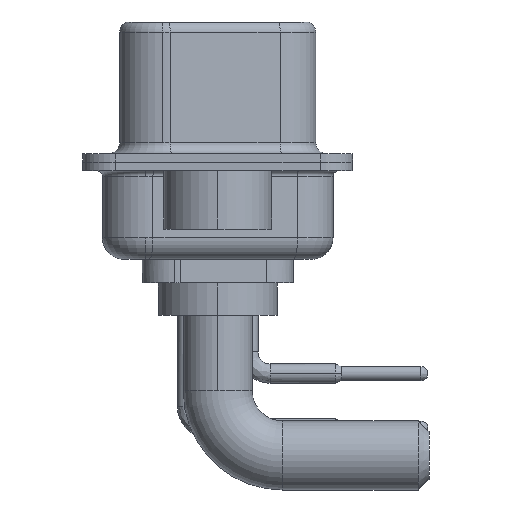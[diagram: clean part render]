
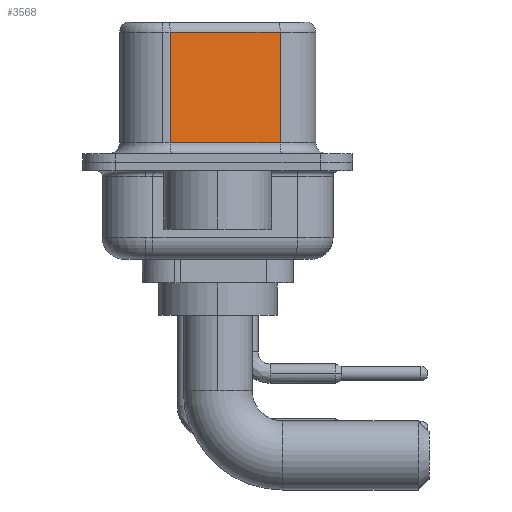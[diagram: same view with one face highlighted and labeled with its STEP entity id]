
A CAD part, left-side view. The second image highlights one B-rep face of the part: STEP entity #3568.
In plain terms, the highlighted planar face has unit normal (-0.985, -0.174, 0).
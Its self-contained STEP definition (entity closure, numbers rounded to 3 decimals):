
#472 = LINE ( 'NONE', #6943, #4627 ) ;
#768 = CARTESIAN_POINT ( 'NONE',  ( 4.555, -2.897, 0.9 ) ) ;
#1092 = EDGE_CURVE ( 'NONE', #7375, #6621, #2627, .T. ) ;
#1129 = EDGE_CURVE ( 'NONE', #11883, #6621, #8667, .T. ) ;
#2255 = EDGE_CURVE ( 'NONE', #7375, #4635, #472, .T. ) ;
#2420 = DIRECTION ( 'NONE',  ( 0.174, -0.985, 0. ) ) ;
#2627 = LINE ( 'NONE', #10373, #11098 ) ;
#2667 = CARTESIAN_POINT ( 'NONE',  ( 3.655, 2.203, 6.02 ) ) ;
#3568 = ADVANCED_FACE ( 'NONE', ( #19395 ), #8153, .F. ) ;
#3642 = VECTOR ( 'NONE', #2420, 1000. ) ;
#3896 = AXIS2_PLACEMENT_3D ( 'NONE', #13359, #6665, #5076 ) ;
#4627 = VECTOR ( 'NONE', #19886, 1000. ) ;
#4635 = VERTEX_POINT ( 'NONE', #2667 ) ;
#5076 = DIRECTION ( 'NONE',  ( -0.174, 0.985, 0. ) ) ;
#5799 = ORIENTED_EDGE ( 'NONE', *, *, #1092, .F. ) ;
#6621 = VERTEX_POINT ( 'NONE', #768 ) ;
#6665 = DIRECTION ( 'NONE',  ( 0.985, 0.174, 0. ) ) ;
#6943 = CARTESIAN_POINT ( 'NONE',  ( 4.555, -2.897, 6.02 ) ) ;
#7375 = VERTEX_POINT ( 'NONE', #19601 ) ;
#7663 = LINE ( 'NONE', #14138, #11700 ) ;
#8153 = PLANE ( 'NONE',  #3896 ) ;
#8667 = LINE ( 'NONE', #16954, #3642 ) ;
#9161 = EDGE_LOOP ( 'NONE', ( #5799, #14070, #19147, #10187 ) ) ;
#10187 = ORIENTED_EDGE ( 'NONE', *, *, #1129, .T. ) ;
#10373 = CARTESIAN_POINT ( 'NONE',  ( 4.555, -2.897, 6.52 ) ) ;
#11098 = VECTOR ( 'NONE', #15267, 1000. ) ;
#11700 = VECTOR ( 'NONE', #12563, 1000. ) ;
#11883 = VERTEX_POINT ( 'NONE', #15766 ) ;
#12563 = DIRECTION ( 'NONE',  ( 0., 0., -1. ) ) ;
#13359 = CARTESIAN_POINT ( 'NONE',  ( 4.555, -2.897, 6.52 ) ) ;
#14070 = ORIENTED_EDGE ( 'NONE', *, *, #2255, .T. ) ;
#14138 = CARTESIAN_POINT ( 'NONE',  ( 3.655, 2.203, 6.52 ) ) ;
#15267 = DIRECTION ( 'NONE',  ( 0., 0., -1. ) ) ;
#15766 = CARTESIAN_POINT ( 'NONE',  ( 3.655, 2.203, 0.9 ) ) ;
#16128 = EDGE_CURVE ( 'NONE', #4635, #11883, #7663, .T. ) ;
#16954 = CARTESIAN_POINT ( 'NONE',  ( 4.555, -2.897, 0.9 ) ) ;
#19147 = ORIENTED_EDGE ( 'NONE', *, *, #16128, .T. ) ;
#19395 = FACE_OUTER_BOUND ( 'NONE', #9161, .T. ) ;
#19601 = CARTESIAN_POINT ( 'NONE',  ( 4.555, -2.897, 6.02 ) ) ;
#19886 = DIRECTION ( 'NONE',  ( -0.174, 0.985, 0. ) ) ;
